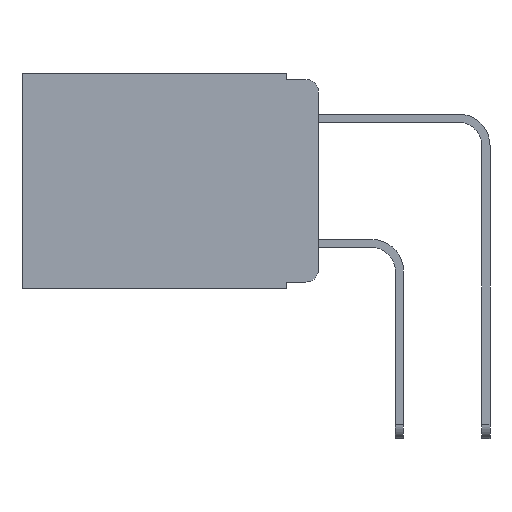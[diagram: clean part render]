
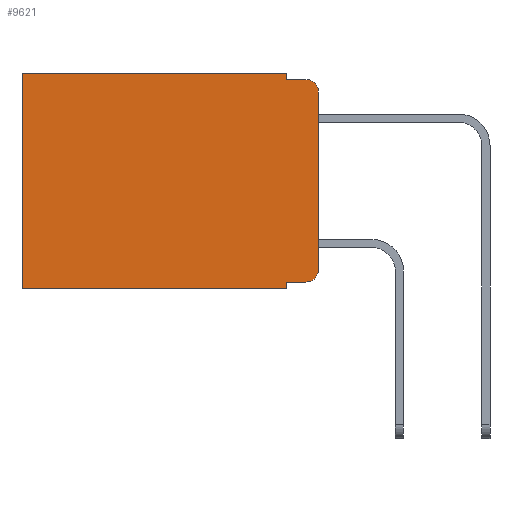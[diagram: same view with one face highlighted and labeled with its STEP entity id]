
A CAD part, left-side view. The second image highlights one B-rep face of the part: STEP entity #9621.
In plain terms, the highlighted planar face has unit normal (-1, 0, 0).
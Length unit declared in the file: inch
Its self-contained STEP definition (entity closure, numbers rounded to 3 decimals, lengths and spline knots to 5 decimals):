
#120 = DIRECTION ( 'NONE',  ( 0., 0., -1. ) ) ;
#226 = CIRCLE ( 'NONE', #6148, 0.02 ) ;
#569 = DIRECTION ( 'NONE',  ( 0., 0., -1. ) ) ;
#693 = EDGE_LOOP ( 'NONE', ( #9124, #11773, #11371, #3752, #9441, #2153, #10289, #3633, #3319, #5856 ) ) ;
#749 = CARTESIAN_POINT ( 'NONE',  ( 0.298, 0., -0.313 ) ) ;
#855 = VERTEX_POINT ( 'NONE', #7306 ) ;
#894 = DIRECTION ( 'NONE',  ( 0., 0., -1. ) ) ;
#943 = VECTOR ( 'NONE', #5274, 39.37008 ) ;
#1313 = VERTEX_POINT ( 'NONE', #12141 ) ;
#1517 = DIRECTION ( 'NONE',  ( 0., -1., 0. ) ) ;
#1550 = LINE ( 'NONE', #2746, #9147 ) ;
#2153 = ORIENTED_EDGE ( 'NONE', *, *, #8114, .T. ) ;
#2298 = VECTOR ( 'NONE', #569, 39.37008 ) ;
#2400 = LINE ( 'NONE', #11233, #7963 ) ;
#2746 = CARTESIAN_POINT ( 'NONE',  ( 0.298, 0., 0. ) ) ;
#2897 = VECTOR ( 'NONE', #6250, 39.37008 ) ;
#3086 = LINE ( 'NONE', #8446, #11212 ) ;
#3173 = DIRECTION ( 'NONE',  ( 1., 0., 0. ) ) ;
#3319 = ORIENTED_EDGE ( 'NONE', *, *, #5465, .T. ) ;
#3353 = LINE ( 'NONE', #11144, #943 ) ;
#3515 = EDGE_CURVE ( 'NONE', #1313, #6627, #226, .T. ) ;
#3625 = VERTEX_POINT ( 'NONE', #8274 ) ;
#3633 = ORIENTED_EDGE ( 'NONE', *, *, #6109, .F. ) ;
#3752 = ORIENTED_EDGE ( 'NONE', *, *, #8793, .F. ) ;
#3857 = EDGE_CURVE ( 'NONE', #12397, #6627, #1550, .T. ) ;
#4285 = VERTEX_POINT ( 'NONE', #9555 ) ;
#4396 = DIRECTION ( 'NONE',  ( 0., 0., -1. ) ) ;
#4571 = DIRECTION ( 'NONE',  ( 0., 1., 0. ) ) ;
#4610 = CARTESIAN_POINT ( 'NONE',  ( 0.298, 0., 0. ) ) ;
#4861 = VECTOR ( 'NONE', #4883, 39.37008 ) ;
#4883 = DIRECTION ( 'NONE',  ( 0., -1., 0. ) ) ;
#4929 = LINE ( 'NONE', #7555, #2298 ) ;
#5193 = LINE ( 'NONE', #11159, #2897 ) ;
#5274 = DIRECTION ( 'NONE',  ( 0., 1., 0. ) ) ;
#5465 = EDGE_CURVE ( 'NONE', #6728, #1313, #3086, .T. ) ;
#5609 = FACE_OUTER_BOUND ( 'NONE', #693, .T. ) ;
#5856 = ORIENTED_EDGE ( 'NONE', *, *, #3515, .T. ) ;
#6109 = EDGE_CURVE ( 'NONE', #6728, #855, #4929, .T. ) ;
#6135 = DIRECTION ( 'NONE',  ( -1., 0., 0. ) ) ;
#6148 = AXIS2_PLACEMENT_3D ( 'NONE', #12003, #6135, #120 ) ;
#6250 = DIRECTION ( 'NONE',  ( 0., 0., -1. ) ) ;
#6627 = VERTEX_POINT ( 'NONE', #749 ) ;
#6728 = VERTEX_POINT ( 'NONE', #8870 ) ;
#6824 = DIRECTION ( 'NONE',  ( -1., 0., 0. ) ) ;
#7306 = CARTESIAN_POINT ( 'NONE',  ( 0.298, 0.051, -0.343 ) ) ;
#7439 = CIRCLE ( 'NONE', #10574, 0.02 ) ;
#7465 = LINE ( 'NONE', #10751, #4861 ) ;
#7555 = CARTESIAN_POINT ( 'NONE',  ( 0.298, 0.051, 0. ) ) ;
#7891 = CARTESIAN_POINT ( 'NONE',  ( 0.298, 0.02, -0.01 ) ) ;
#7893 = VERTEX_POINT ( 'NONE', #7891 ) ;
#7956 = CARTESIAN_POINT ( 'NONE',  ( 0.298, 0.051, -0.01 ) ) ;
#7963 = VECTOR ( 'NONE', #4396, 39.37008 ) ;
#8005 = CARTESIAN_POINT ( 'NONE',  ( 0.298, 0., -0.03 ) ) ;
#8114 = EDGE_CURVE ( 'NONE', #4285, #3625, #5193, .T. ) ;
#8274 = CARTESIAN_POINT ( 'NONE',  ( 0.298, 0.473, -0.343 ) ) ;
#8314 = EDGE_CURVE ( 'NONE', #12279, #4285, #10862, .T. ) ;
#8446 = CARTESIAN_POINT ( 'NONE',  ( 0.298, 0.051, -0.333 ) ) ;
#8718 = EDGE_CURVE ( 'NONE', #855, #3625, #3353, .T. ) ;
#8793 = EDGE_CURVE ( 'NONE', #12279, #10799, #2400, .T. ) ;
#8804 = CARTESIAN_POINT ( 'NONE',  ( 0.298, 0.051, 0. ) ) ;
#8870 = CARTESIAN_POINT ( 'NONE',  ( 0.298, 0.051, -0.333 ) ) ;
#9063 = CARTESIAN_POINT ( 'NONE',  ( 0.298, 0., 0. ) ) ;
#9124 = ORIENTED_EDGE ( 'NONE', *, *, #3857, .F. ) ;
#9147 = VECTOR ( 'NONE', #10605, 39.37008 ) ;
#9441 = ORIENTED_EDGE ( 'NONE', *, *, #8314, .T. ) ;
#9448 = EDGE_CURVE ( 'NONE', #10799, #7893, #7465, .T. ) ;
#9555 = CARTESIAN_POINT ( 'NONE',  ( 0.298, 0.473, 0. ) ) ;
#9621 = ADVANCED_FACE ( 'NONE', ( #5609 ), #11920, .F. ) ;
#10043 = DIRECTION ( 'NONE',  ( 0., 0., -1. ) ) ;
#10289 = ORIENTED_EDGE ( 'NONE', *, *, #8718, .F. ) ;
#10574 = AXIS2_PLACEMENT_3D ( 'NONE', #12693, #6824, #894 ) ;
#10605 = DIRECTION ( 'NONE',  ( 0., 0., -1. ) ) ;
#10724 = EDGE_CURVE ( 'NONE', #12397, #7893, #7439, .T. ) ;
#10751 = CARTESIAN_POINT ( 'NONE',  ( 0.298, 0.051, -0.01 ) ) ;
#10799 = VERTEX_POINT ( 'NONE', #7956 ) ;
#10862 = LINE ( 'NONE', #4610, #12812 ) ;
#10885 = AXIS2_PLACEMENT_3D ( 'NONE', #9063, #3173, #10043 ) ;
#11144 = CARTESIAN_POINT ( 'NONE',  ( 0.298, 0., -0.343 ) ) ;
#11159 = CARTESIAN_POINT ( 'NONE',  ( 0.298, 0.473, 0. ) ) ;
#11212 = VECTOR ( 'NONE', #1517, 39.37008 ) ;
#11233 = CARTESIAN_POINT ( 'NONE',  ( 0.298, 0.051, 0. ) ) ;
#11371 = ORIENTED_EDGE ( 'NONE', *, *, #9448, .F. ) ;
#11773 = ORIENTED_EDGE ( 'NONE', *, *, #10724, .T. ) ;
#11920 = PLANE ( 'NONE',  #10885 ) ;
#12003 = CARTESIAN_POINT ( 'NONE',  ( 0.298, 0.02, -0.313 ) ) ;
#12141 = CARTESIAN_POINT ( 'NONE',  ( 0.298, 0.02, -0.333 ) ) ;
#12279 = VERTEX_POINT ( 'NONE', #8804 ) ;
#12397 = VERTEX_POINT ( 'NONE', #8005 ) ;
#12693 = CARTESIAN_POINT ( 'NONE',  ( 0.298, 0.02, -0.03 ) ) ;
#12812 = VECTOR ( 'NONE', #4571, 39.37008 ) ;
